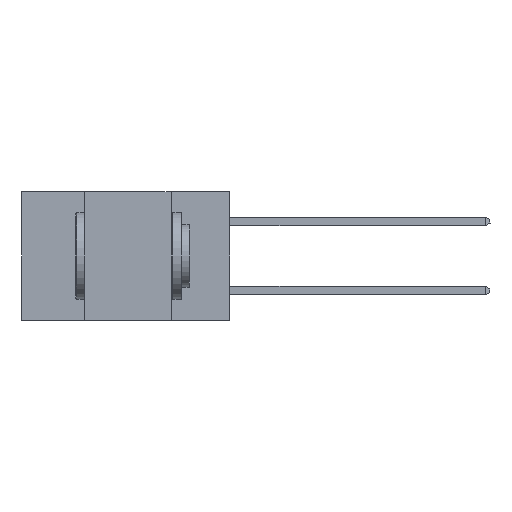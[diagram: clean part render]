
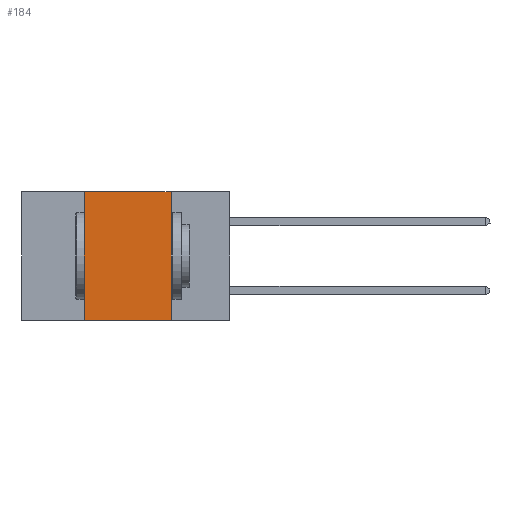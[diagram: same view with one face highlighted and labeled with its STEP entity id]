
A CAD part, left-side view. The second image highlights one B-rep face of the part: STEP entity #184.
In plain terms, the highlighted planar face has unit normal (-1, 0, 0).
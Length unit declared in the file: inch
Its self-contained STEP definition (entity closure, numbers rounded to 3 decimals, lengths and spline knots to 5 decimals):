
#184 = ADVANCED_FACE ( 'NONE', ( #29027 ), #15000, .F. ) ;
#275 = DIRECTION ( 'NONE',  ( 0., -1., 0. ) ) ;
#568 = DIRECTION ( 'NONE',  ( 0., 0., 1. ) ) ;
#627 = CARTESIAN_POINT ( 'NONE',  ( 0., 0.6, 0. ) ) ;
#2441 = LINE ( 'NONE', #9636, #4594 ) ;
#2943 = DIRECTION ( 'NONE',  ( 0., -1., 0. ) ) ;
#3046 = CARTESIAN_POINT ( 'NONE',  ( 0., 0.42, 0. ) ) ;
#4285 = LINE ( 'NONE', #7003, #24536 ) ;
#4588 = VERTEX_POINT ( 'NONE', #23205 ) ;
#4594 = VECTOR ( 'NONE', #568, 39.37008 ) ;
#4860 = ORIENTED_EDGE ( 'NONE', *, *, #18499, .T. ) ;
#4875 = VECTOR ( 'NONE', #12361, 39.37008 ) ;
#6853 = VERTEX_POINT ( 'NONE', #25124 ) ;
#7003 = CARTESIAN_POINT ( 'NONE',  ( 0., 0.6, -0.37 ) ) ;
#7428 = VERTEX_POINT ( 'NONE', #15026 ) ;
#9636 = CARTESIAN_POINT ( 'NONE',  ( 0., 0.42, 0. ) ) ;
#10167 = CARTESIAN_POINT ( 'NONE',  ( 0., 0.6, 0. ) ) ;
#11366 = ORIENTED_EDGE ( 'NONE', *, *, #15958, .F. ) ;
#12096 = ORIENTED_EDGE ( 'NONE', *, *, #20315, .F. ) ;
#12361 = DIRECTION ( 'NONE',  ( 0., 0., -1. ) ) ;
#14707 = DIRECTION ( 'NONE',  ( 1., 0., 0. ) ) ;
#15000 = PLANE ( 'NONE',  #28045 ) ;
#15026 = CARTESIAN_POINT ( 'NONE',  ( 0., 0.17, 0. ) ) ;
#15958 = EDGE_CURVE ( 'NONE', #21286, #7428, #23947, .T. ) ;
#18499 = EDGE_CURVE ( 'NONE', #6853, #4588, #4285, .T. ) ;
#19066 = EDGE_CURVE ( 'NONE', #6853, #21286, #2441, .T. ) ;
#19241 = CARTESIAN_POINT ( 'NONE',  ( 0., 0.17, 0. ) ) ;
#19476 = DIRECTION ( 'NONE',  ( 0., 0., -1. ) ) ;
#20315 = EDGE_CURVE ( 'NONE', #7428, #4588, #29531, .T. ) ;
#20581 = ORIENTED_EDGE ( 'NONE', *, *, #19066, .F. ) ;
#21286 = VERTEX_POINT ( 'NONE', #3046 ) ;
#23205 = CARTESIAN_POINT ( 'NONE',  ( 0., 0.17, -0.37 ) ) ;
#23947 = LINE ( 'NONE', #627, #25412 ) ;
#24536 = VECTOR ( 'NONE', #275, 39.37008 ) ;
#25124 = CARTESIAN_POINT ( 'NONE',  ( 0., 0.42, -0.37 ) ) ;
#25412 = VECTOR ( 'NONE', #2943, 39.37008 ) ;
#27224 = EDGE_LOOP ( 'NONE', ( #12096, #11366, #20581, #4860 ) ) ;
#28045 = AXIS2_PLACEMENT_3D ( 'NONE', #10167, #14707, #19476 ) ;
#29027 = FACE_OUTER_BOUND ( 'NONE', #27224, .T. ) ;
#29531 = LINE ( 'NONE', #19241, #4875 ) ;
